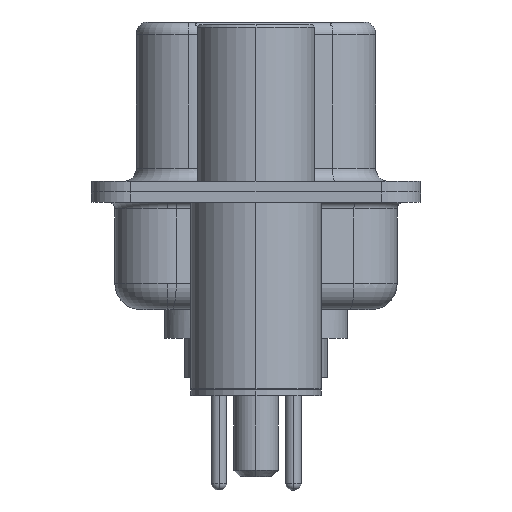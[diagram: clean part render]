
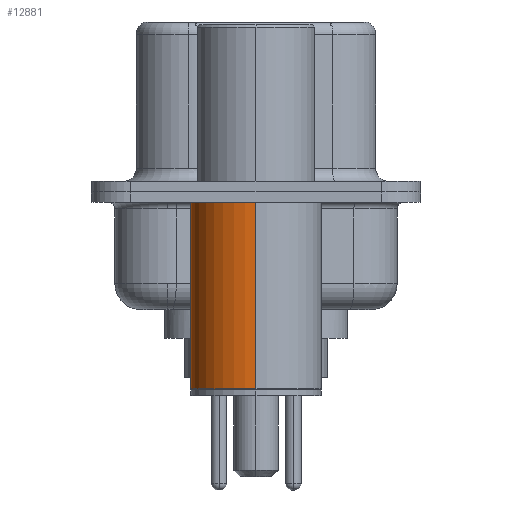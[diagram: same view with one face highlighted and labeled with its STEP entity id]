
A CAD part, left-side view. The second image highlights one B-rep face of the part: STEP entity #12881.
In plain terms, the highlighted cylindrical face has radius 2.5 mm (diameter 5 mm), a partial arc.
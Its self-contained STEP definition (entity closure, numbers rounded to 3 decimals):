
#275 = EDGE_CURVE ( 'NONE', #708, #3178, #6315, .T. ) ;
#629 = CYLINDRICAL_SURFACE ( 'NONE', #12017, 2.5 ) ;
#708 = VERTEX_POINT ( 'NONE', #11563 ) ;
#859 = ORIENTED_EDGE ( 'NONE', *, *, #275, .F. ) ;
#1296 = DIRECTION ( 'NONE',  ( 0., 0., 1. ) ) ;
#1386 = CARTESIAN_POINT ( 'NONE',  ( 0., 0., -7.525 ) ) ;
#1462 = DIRECTION ( 'NONE',  ( 0., 0., 1. ) ) ;
#1624 = CARTESIAN_POINT ( 'NONE',  ( -2.5, 0., -0.4 ) ) ;
#2084 = EDGE_CURVE ( 'NONE', #17704, #19721, #11578, .T. ) ;
#2466 = VECTOR ( 'NONE', #16982, 1000. ) ;
#2953 = VECTOR ( 'NONE', #9835, 1000. ) ;
#3099 = DIRECTION ( 'NONE',  ( 1., 0., 0. ) ) ;
#3161 = EDGE_CURVE ( 'NONE', #708, #17704, #5717, .T. ) ;
#3178 = VERTEX_POINT ( 'NONE', #17619 ) ;
#3896 = DIRECTION ( 'NONE',  ( 1., 0., 0. ) ) ;
#4161 = AXIS2_PLACEMENT_3D ( 'NONE', #9497, #20888, #11121 ) ;
#5717 = CIRCLE ( 'NONE', #12498, 2.5 ) ;
#6315 = LINE ( 'NONE', #14145, #2466 ) ;
#6386 = CARTESIAN_POINT ( 'NONE',  ( 0., 0., 0.581 ) ) ;
#7781 = EDGE_LOOP ( 'NONE', ( #8516, #12028, #19673, #859 ) ) ;
#8516 = ORIENTED_EDGE ( 'NONE', *, *, #3161, .T. ) ;
#9497 = CARTESIAN_POINT ( 'NONE',  ( 0., 0., -0.4 ) ) ;
#9808 = CARTESIAN_POINT ( 'NONE',  ( -2.5, 0., -7.525 ) ) ;
#9835 = DIRECTION ( 'NONE',  ( 0., 0., 1. ) ) ;
#11121 = DIRECTION ( 'NONE',  ( 1., 0., 0. ) ) ;
#11563 = CARTESIAN_POINT ( 'NONE',  ( 2.5, 0., -7.525 ) ) ;
#11578 = LINE ( 'NONE', #11743, #2953 ) ;
#11743 = CARTESIAN_POINT ( 'NONE',  ( -2.5, 0., 0.581 ) ) ;
#12017 = AXIS2_PLACEMENT_3D ( 'NONE', #6386, #1462, #3099 ) ;
#12028 = ORIENTED_EDGE ( 'NONE', *, *, #2084, .T. ) ;
#12275 = EDGE_CURVE ( 'NONE', #3178, #19721, #19488, .T. ) ;
#12498 = AXIS2_PLACEMENT_3D ( 'NONE', #1386, #1296, #3896 ) ;
#12881 = ADVANCED_FACE ( 'NONE', ( #13545 ), #629, .T. ) ;
#13545 = FACE_OUTER_BOUND ( 'NONE', #7781, .T. ) ;
#14145 = CARTESIAN_POINT ( 'NONE',  ( 2.5, 0., 0.581 ) ) ;
#16982 = DIRECTION ( 'NONE',  ( 0., 0., 1. ) ) ;
#17619 = CARTESIAN_POINT ( 'NONE',  ( 2.5, 0., -0.4 ) ) ;
#17704 = VERTEX_POINT ( 'NONE', #9808 ) ;
#19488 = CIRCLE ( 'NONE', #4161, 2.5 ) ;
#19673 = ORIENTED_EDGE ( 'NONE', *, *, #12275, .F. ) ;
#19721 = VERTEX_POINT ( 'NONE', #1624 ) ;
#20888 = DIRECTION ( 'NONE',  ( 0., 0., 1. ) ) ;
